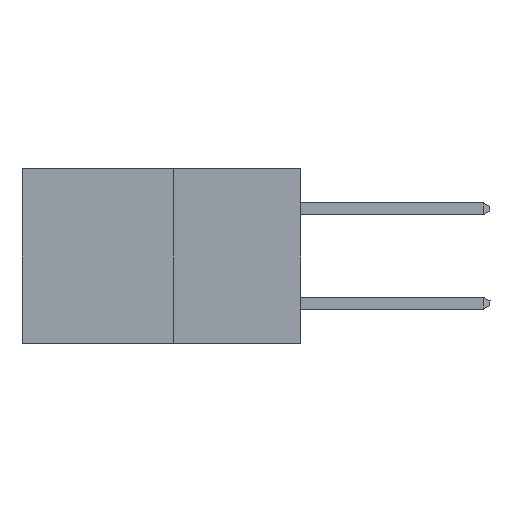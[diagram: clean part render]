
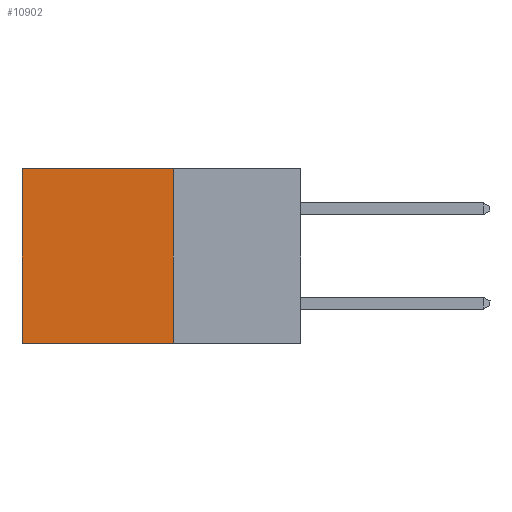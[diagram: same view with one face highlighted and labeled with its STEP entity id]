
A CAD part, left-side view. The second image highlights one B-rep face of the part: STEP entity #10902.
In plain terms, the highlighted planar face has unit normal (-1, 0, 0).
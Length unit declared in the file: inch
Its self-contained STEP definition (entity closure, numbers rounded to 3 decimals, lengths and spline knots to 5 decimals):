
#675 = VERTEX_POINT ( 'NONE', #24056 ) ;
#1024 = VERTEX_POINT ( 'NONE', #9599 ) ;
#3461 = AXIS2_PLACEMENT_3D ( 'NONE', #22356, #24605, #10973 ) ;
#3501 = DIRECTION ( 'NONE',  ( 0., 1., 0. ) ) ;
#4730 = CARTESIAN_POINT ( 'NONE',  ( 0.277, 0.27, -0.37 ) ) ;
#7507 = VECTOR ( 'NONE', #25366, 39.37008 ) ;
#8702 = VERTEX_POINT ( 'NONE', #25383 ) ;
#9252 = VECTOR ( 'NONE', #3501, 39.37008 ) ;
#9352 = CARTESIAN_POINT ( 'NONE',  ( 0.277, 0.27, 0. ) ) ;
#9599 = CARTESIAN_POINT ( 'NONE',  ( 0.277, 0.27, 0. ) ) ;
#9968 = LINE ( 'NONE', #12678, #9252 ) ;
#10902 = ADVANCED_FACE ( 'NONE', ( #12200 ), #17765, .F. ) ;
#10973 = DIRECTION ( 'NONE',  ( 0., 0., -1. ) ) ;
#11739 = EDGE_CURVE ( 'NONE', #1024, #25531, #13597, .T. ) ;
#12036 = LINE ( 'NONE', #4730, #22756 ) ;
#12200 = FACE_OUTER_BOUND ( 'NONE', #19353, .T. ) ;
#12678 = CARTESIAN_POINT ( 'NONE',  ( 0.277, 0.27, -0.37 ) ) ;
#13435 = ORIENTED_EDGE ( 'NONE', *, *, #11739, .T. ) ;
#13597 = LINE ( 'NONE', #9352, #7507 ) ;
#15717 = CARTESIAN_POINT ( 'NONE',  ( 0.277, 0.59, -0.37 ) ) ;
#15803 = VECTOR ( 'NONE', #20286, 39.37008 ) ;
#17765 = PLANE ( 'NONE',  #3461 ) ;
#19339 = EDGE_CURVE ( 'NONE', #25531, #8702, #21861, .T. ) ;
#19353 = EDGE_LOOP ( 'NONE', ( #21650, #25177, #22988, #13435 ) ) ;
#20286 = DIRECTION ( 'NONE',  ( 0., 0., -1. ) ) ;
#21650 = ORIENTED_EDGE ( 'NONE', *, *, #19339, .T. ) ;
#21861 = LINE ( 'NONE', #15717, #15803 ) ;
#22356 = CARTESIAN_POINT ( 'NONE',  ( 0.277, 0.27, -0.37 ) ) ;
#22727 = EDGE_CURVE ( 'NONE', #675, #8702, #9968, .T. ) ;
#22756 = VECTOR ( 'NONE', #23037, 39.37008 ) ;
#22988 = ORIENTED_EDGE ( 'NONE', *, *, #26487, .F. ) ;
#23037 = DIRECTION ( 'NONE',  ( 0., 0., -1. ) ) ;
#24056 = CARTESIAN_POINT ( 'NONE',  ( 0.277, 0.27, -0.37 ) ) ;
#24605 = DIRECTION ( 'NONE',  ( 1., 0., 0. ) ) ;
#25177 = ORIENTED_EDGE ( 'NONE', *, *, #22727, .F. ) ;
#25366 = DIRECTION ( 'NONE',  ( 0., 1., 0. ) ) ;
#25383 = CARTESIAN_POINT ( 'NONE',  ( 0.277, 0.59, -0.37 ) ) ;
#25531 = VERTEX_POINT ( 'NONE', #27656 ) ;
#26487 = EDGE_CURVE ( 'NONE', #1024, #675, #12036, .T. ) ;
#27656 = CARTESIAN_POINT ( 'NONE',  ( 0.277, 0.59, 0. ) ) ;
